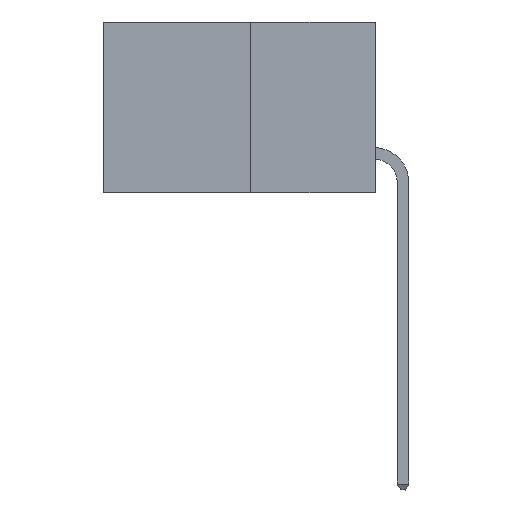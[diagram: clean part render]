
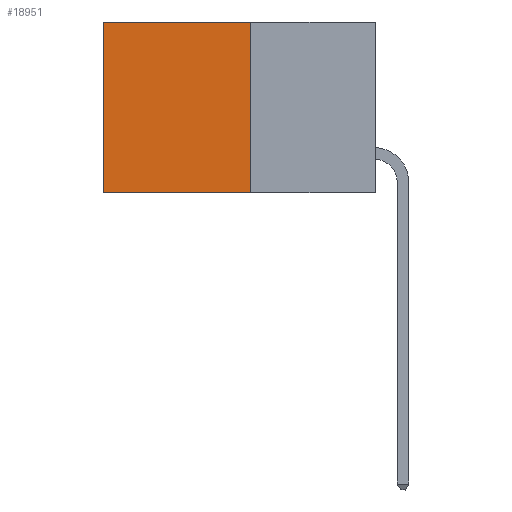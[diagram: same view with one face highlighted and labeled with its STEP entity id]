
A CAD part, left-side view. The second image highlights one B-rep face of the part: STEP entity #18951.
In plain terms, the highlighted planar face has unit normal (-1, 0, 0).
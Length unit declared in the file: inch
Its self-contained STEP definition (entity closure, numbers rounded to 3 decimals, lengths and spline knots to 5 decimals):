
#152 = VECTOR ( 'NONE', #12100, 39.37008 ) ;
#970 = AXIS2_PLACEMENT_3D ( 'NONE', #12924, #3599, #14427 ) ;
#1005 = EDGE_CURVE ( 'NONE', #5663, #2636, #5491, .T. ) ;
#1173 = FACE_OUTER_BOUND ( 'NONE', #9833, .T. ) ;
#2027 = PLANE ( 'NONE',  #970 ) ;
#2253 = DIRECTION ( 'NONE',  ( 0., 0., -1. ) ) ;
#2636 = VERTEX_POINT ( 'NONE', #7086 ) ;
#3599 = DIRECTION ( 'NONE',  ( 1., 0., 0. ) ) ;
#3811 = LINE ( 'NONE', #8080, #7494 ) ;
#5068 = ORIENTED_EDGE ( 'NONE', *, *, #1005, .T. ) ;
#5111 = ORIENTED_EDGE ( 'NONE', *, *, #7515, .F. ) ;
#5426 = ORIENTED_EDGE ( 'NONE', *, *, #6963, .F. ) ;
#5491 = LINE ( 'NONE', #8064, #12760 ) ;
#5549 = VERTEX_POINT ( 'NONE', #10132 ) ;
#5650 = ORIENTED_EDGE ( 'NONE', *, *, #6012, .T. ) ;
#5663 = VERTEX_POINT ( 'NONE', #12400 ) ;
#6012 = EDGE_CURVE ( 'NONE', #6231, #5663, #3811, .T. ) ;
#6231 = VERTEX_POINT ( 'NONE', #7719 ) ;
#6963 = EDGE_CURVE ( 'NONE', #6231, #5549, #10926, .T. ) ;
#7086 = CARTESIAN_POINT ( 'NONE',  ( 0.277, 0.59, -0.37 ) ) ;
#7494 = VECTOR ( 'NONE', #8153, 39.37008 ) ;
#7515 = EDGE_CURVE ( 'NONE', #5549, #2636, #16664, .T. ) ;
#7719 = CARTESIAN_POINT ( 'NONE',  ( 0.277, 0.27, 0. ) ) ;
#8064 = CARTESIAN_POINT ( 'NONE',  ( 0.277, 0.59, -0.37 ) ) ;
#8080 = CARTESIAN_POINT ( 'NONE',  ( 0.277, 0.27, 0. ) ) ;
#8153 = DIRECTION ( 'NONE',  ( 0., 1., 0. ) ) ;
#9833 = EDGE_LOOP ( 'NONE', ( #5068, #5111, #5426, #5650 ) ) ;
#10132 = CARTESIAN_POINT ( 'NONE',  ( 0.277, 0.27, -0.37 ) ) ;
#10628 = CARTESIAN_POINT ( 'NONE',  ( 0.277, 0.27, -0.37 ) ) ;
#10926 = LINE ( 'NONE', #19894, #14444 ) ;
#12100 = DIRECTION ( 'NONE',  ( 0., 1., 0. ) ) ;
#12400 = CARTESIAN_POINT ( 'NONE',  ( 0.277, 0.59, 0. ) ) ;
#12760 = VECTOR ( 'NONE', #17993, 39.37008 ) ;
#12924 = CARTESIAN_POINT ( 'NONE',  ( 0.277, 0.27, -0.37 ) ) ;
#14427 = DIRECTION ( 'NONE',  ( 0., 0., -1. ) ) ;
#14444 = VECTOR ( 'NONE', #2253, 39.37008 ) ;
#16664 = LINE ( 'NONE', #10628, #152 ) ;
#17993 = DIRECTION ( 'NONE',  ( 0., 0., -1. ) ) ;
#18951 = ADVANCED_FACE ( 'NONE', ( #1173 ), #2027, .F. ) ;
#19894 = CARTESIAN_POINT ( 'NONE',  ( 0.277, 0.27, -0.37 ) ) ;
